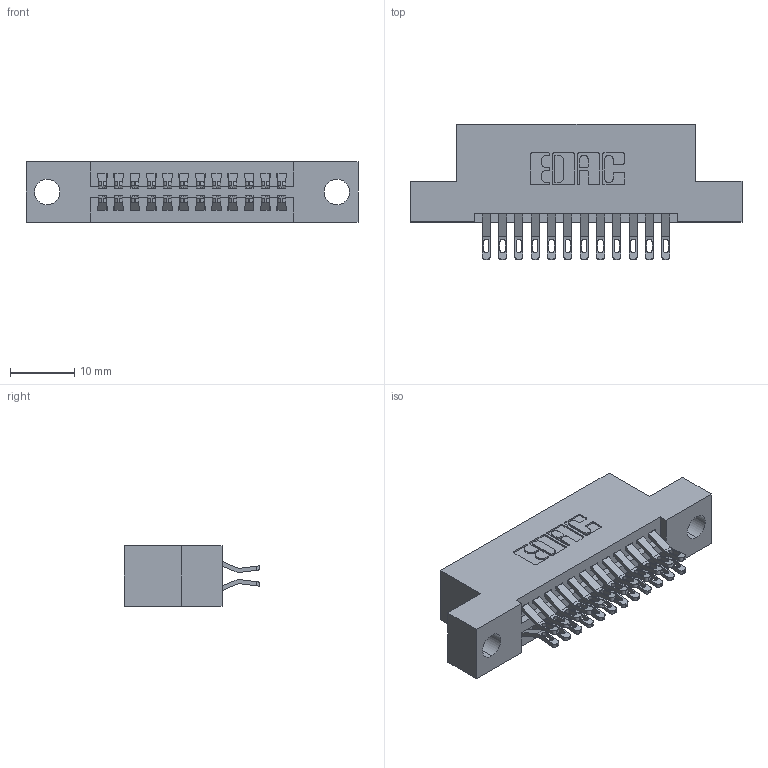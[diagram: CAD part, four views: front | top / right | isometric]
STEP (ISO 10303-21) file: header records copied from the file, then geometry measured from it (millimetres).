
FILE_DESCRIPTION (( 'STEP AP203' ), '1' );
FILE_NAME ('395-024-555-204.STEP', '2021-06-16T19:15:27', ( '' ), ( '' ), 'SwSTEP 2.0', 'SolidWorks 2020', '' );
FILE_SCHEMA (( 'CONFIG_CONTROL_DESIGN' ));
Length unit declared in the file: inch
Products named in the file (3): 395-024-555-204; 345 Part_Flush Mounting Lugs - 0.156 Dia-TI; 345-292-001_555 Tail
Assembly tree (25 placements, depth 2):
  395-024-555-204
    345 Part_Flush Mounting Lugs - 0.156 Dia-TI
    345-292-001_555 Tail  x24
Bounding box: 51.69 x 21.13 x 9.4 mm (x, y, z)
Volume: 4706.3 mm3; surface area: 6469.4 mm2
Topology: 25 solids, 25 shells, 1484 faces, 4625 edges, 3082 vertices
Faces by surface type: plane 838, cylinder 646
Entity records: 14199 total; most frequent: CARTESIAN_POINT 2448, ORIENTED_EDGE 2350, DIRECTION 2163, EDGE_CURVE 1175, VECTOR 975, LINE 975, VERTEX_POINT 782, AXIS2_PLACEMENT_3D 594
